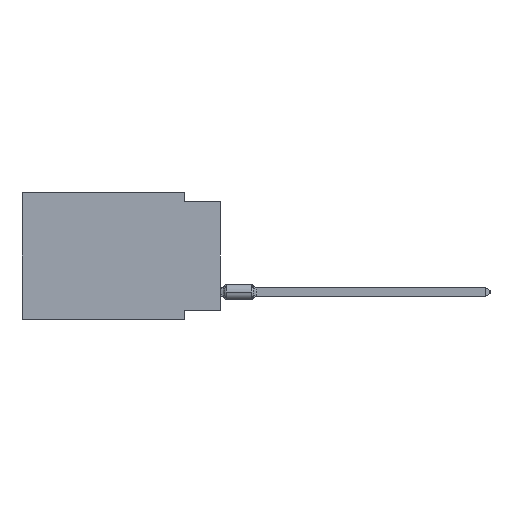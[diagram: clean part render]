
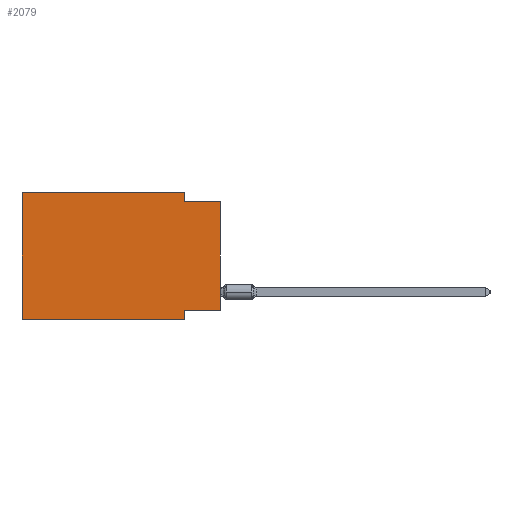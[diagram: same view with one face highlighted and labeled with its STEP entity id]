
A CAD part, left-side view. The second image highlights one B-rep face of the part: STEP entity #2079.
In plain terms, the highlighted planar face has unit normal (-1, 0, 0).
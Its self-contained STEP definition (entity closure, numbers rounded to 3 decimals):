
#255 = ORIENTED_EDGE ( 'NONE', *, *, #43681, .F. ) ;
#2079 = ADVANCED_FACE ( 'NONE', ( #48709 ), #34810, .F. ) ;
#3198 = DIRECTION ( 'NONE',  ( 0., 0., 1. ) ) ;
#3783 = ORIENTED_EDGE ( 'NONE', *, *, #41329, .F. ) ;
#4385 = EDGE_CURVE ( 'NONE', #41870, #9713, #59750, .T. ) ;
#5314 = VECTOR ( 'NONE', #28306, 1000. ) ;
#6229 = VECTOR ( 'NONE', #52321, 1000. ) ;
#6689 = LINE ( 'NONE', #56015, #16184 ) ;
#7894 = CARTESIAN_POINT ( 'NONE',  ( 0., 0., -0.635 ) ) ;
#8635 = LINE ( 'NONE', #21980, #39971 ) ;
#8970 = LINE ( 'NONE', #22327, #10365 ) ;
#9517 = ORIENTED_EDGE ( 'NONE', *, *, #29878, .T. ) ;
#9713 = VERTEX_POINT ( 'NONE', #39632 ) ;
#10365 = VECTOR ( 'NONE', #49839, 1000. ) ;
#14580 = DIRECTION ( 'NONE',  ( 0., 1., 0. ) ) ;
#16184 = VECTOR ( 'NONE', #14580, 1000. ) ;
#17540 = CARTESIAN_POINT ( 'NONE',  ( 0., 13.97, 0. ) ) ;
#18302 = DIRECTION ( 'NONE',  ( 0., -1., 0. ) ) ;
#18308 = ORIENTED_EDGE ( 'NONE', *, *, #29771, .F. ) ;
#18980 = ORIENTED_EDGE ( 'NONE', *, *, #46683, .F. ) ;
#19903 = VECTOR ( 'NONE', #22690, 1000. ) ;
#20150 = CARTESIAN_POINT ( 'NONE',  ( 0., 0., -8.255 ) ) ;
#20372 = CARTESIAN_POINT ( 'NONE',  ( 0., 13.97, -8.89 ) ) ;
#20898 = DIRECTION ( 'NONE',  ( 1., 0., 0. ) ) ;
#21980 = CARTESIAN_POINT ( 'NONE',  ( 0., 13.97, 0. ) ) ;
#22327 = CARTESIAN_POINT ( 'NONE',  ( 0., 0., 0. ) ) ;
#22690 = DIRECTION ( 'NONE',  ( 0., 0., -1. ) ) ;
#27024 = VECTOR ( 'NONE', #52650, 1000. ) ;
#28306 = DIRECTION ( 'NONE',  ( 0., 0., -1. ) ) ;
#29034 = CARTESIAN_POINT ( 'NONE',  ( 0., 0., -0.635 ) ) ;
#29058 = CARTESIAN_POINT ( 'NONE',  ( 0., 2.54, -0.635 ) ) ;
#29661 = EDGE_LOOP ( 'NONE', ( #9517, #36303, #3783, #52313, #18980, #30255, #255, #18308 ) ) ;
#29771 = EDGE_CURVE ( 'NONE', #53642, #55063, #6689, .T. ) ;
#29878 = EDGE_CURVE ( 'NONE', #53642, #44609, #8970, .T. ) ;
#30255 = ORIENTED_EDGE ( 'NONE', *, *, #4385, .T. ) ;
#31598 = CARTESIAN_POINT ( 'NONE',  ( 0., 13.97, 0. ) ) ;
#32250 = LINE ( 'NONE', #36489, #5314 ) ;
#33104 = CARTESIAN_POINT ( 'NONE',  ( 0., 13.97, -8.89 ) ) ;
#34208 = LINE ( 'NONE', #58617, #27024 ) ;
#34810 = PLANE ( 'NONE',  #40847 ) ;
#36303 = ORIENTED_EDGE ( 'NONE', *, *, #47776, .F. ) ;
#36489 = CARTESIAN_POINT ( 'NONE',  ( 0., 2.54, 0. ) ) ;
#36984 = EDGE_CURVE ( 'NONE', #42970, #42680, #34208, .T. ) ;
#38052 = CARTESIAN_POINT ( 'NONE',  ( 0., 2.54, 0. ) ) ;
#38103 = LINE ( 'NONE', #29034, #6229 ) ;
#39632 = CARTESIAN_POINT ( 'NONE',  ( 0., 2.54, -8.89 ) ) ;
#39971 = VECTOR ( 'NONE', #3198, 1000. ) ;
#40847 = AXIS2_PLACEMENT_3D ( 'NONE', #17540, #20898, #49326 ) ;
#41329 = EDGE_CURVE ( 'NONE', #42680, #42234, #32250, .T. ) ;
#41870 = VERTEX_POINT ( 'NONE', #20372 ) ;
#42234 = VERTEX_POINT ( 'NONE', #29058 ) ;
#42680 = VERTEX_POINT ( 'NONE', #38052 ) ;
#42970 = VERTEX_POINT ( 'NONE', #31598 ) ;
#43681 = EDGE_CURVE ( 'NONE', #55063, #9713, #54159, .T. ) ;
#44609 = VERTEX_POINT ( 'NONE', #7894 ) ;
#46683 = EDGE_CURVE ( 'NONE', #41870, #42970, #8635, .T. ) ;
#47776 = EDGE_CURVE ( 'NONE', #42234, #44609, #38103, .T. ) ;
#48709 = FACE_OUTER_BOUND ( 'NONE', #29661, .T. ) ;
#49326 = DIRECTION ( 'NONE',  ( 0., 0., -1. ) ) ;
#49839 = DIRECTION ( 'NONE',  ( 0., 0., 1. ) ) ;
#52313 = ORIENTED_EDGE ( 'NONE', *, *, #36984, .F. ) ;
#52321 = DIRECTION ( 'NONE',  ( 0., -1., 0. ) ) ;
#52650 = DIRECTION ( 'NONE',  ( 0., -1., 0. ) ) ;
#53642 = VERTEX_POINT ( 'NONE', #20150 ) ;
#54159 = LINE ( 'NONE', #54736, #19903 ) ;
#54736 = CARTESIAN_POINT ( 'NONE',  ( 0., 2.54, -8.89 ) ) ;
#55063 = VERTEX_POINT ( 'NONE', #59757 ) ;
#56015 = CARTESIAN_POINT ( 'NONE',  ( 0., 0., -8.255 ) ) ;
#57156 = VECTOR ( 'NONE', #18302, 1000. ) ;
#58617 = CARTESIAN_POINT ( 'NONE',  ( 0., 13.97, 0. ) ) ;
#59750 = LINE ( 'NONE', #33104, #57156 ) ;
#59757 = CARTESIAN_POINT ( 'NONE',  ( 0., 2.54, -8.255 ) ) ;
